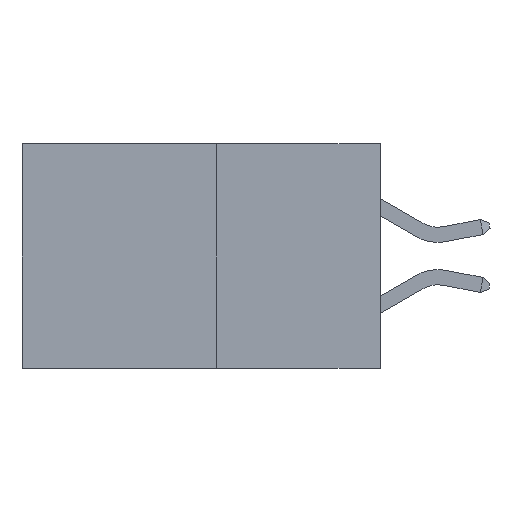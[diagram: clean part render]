
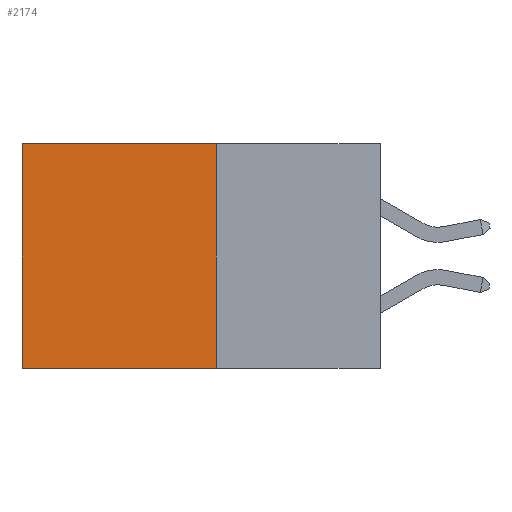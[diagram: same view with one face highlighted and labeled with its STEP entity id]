
A CAD part, left-side view. The second image highlights one B-rep face of the part: STEP entity #2174.
In plain terms, the highlighted planar face has unit normal (-1, 0, 0).
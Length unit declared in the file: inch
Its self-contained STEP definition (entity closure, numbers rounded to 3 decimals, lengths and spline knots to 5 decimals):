
#420 = LINE ( 'NONE', #1278, #32163 ) ;
#1046 = EDGE_CURVE ( 'NONE', #8502, #1778, #3159, .T. ) ;
#1087 = ORIENTED_EDGE ( 'NONE', *, *, #10690, .F. ) ;
#1278 = CARTESIAN_POINT ( 'NONE',  ( 0.277, 0.27, -0.37 ) ) ;
#1484 = PLANE ( 'NONE',  #13002 ) ;
#1778 = VERTEX_POINT ( 'NONE', #25335 ) ;
#2174 = ADVANCED_FACE ( 'NONE', ( #19634 ), #1484, .F. ) ;
#2324 = CARTESIAN_POINT ( 'NONE',  ( 0.277, 0.27, -0.37 ) ) ;
#3159 = LINE ( 'NONE', #20401, #12283 ) ;
#4904 = VECTOR ( 'NONE', #17409, 39.37008 ) ;
#6330 = ORIENTED_EDGE ( 'NONE', *, *, #1046, .T. ) ;
#8502 = VERTEX_POINT ( 'NONE', #27455 ) ;
#8801 = ORIENTED_EDGE ( 'NONE', *, *, #24155, .T. ) ;
#9324 = VECTOR ( 'NONE', #13642, 39.37008 ) ;
#10690 = EDGE_CURVE ( 'NONE', #8502, #12265, #420, .T. ) ;
#11137 = CARTESIAN_POINT ( 'NONE',  ( 0.277, 0.59, -0.37 ) ) ;
#12265 = VERTEX_POINT ( 'NONE', #29933 ) ;
#12283 = VECTOR ( 'NONE', #19959, 39.37008 ) ;
#13002 = AXIS2_PLACEMENT_3D ( 'NONE', #16773, #32307, #31680 ) ;
#13642 = DIRECTION ( 'NONE',  ( 0., 0., -1. ) ) ;
#15832 = ORIENTED_EDGE ( 'NONE', *, *, #20742, .F. ) ;
#16773 = CARTESIAN_POINT ( 'NONE',  ( 0.277, 0.27, -0.37 ) ) ;
#17409 = DIRECTION ( 'NONE',  ( 0., 1., 0. ) ) ;
#17697 = VERTEX_POINT ( 'NONE', #18727 ) ;
#18727 = CARTESIAN_POINT ( 'NONE',  ( 0.277, 0.59, -0.37 ) ) ;
#19634 = FACE_OUTER_BOUND ( 'NONE', #28226, .T. ) ;
#19959 = DIRECTION ( 'NONE',  ( 0., 1., 0. ) ) ;
#20401 = CARTESIAN_POINT ( 'NONE',  ( 0.277, 0.27, 0. ) ) ;
#20742 = EDGE_CURVE ( 'NONE', #12265, #17697, #24153, .T. ) ;
#21435 = DIRECTION ( 'NONE',  ( 0., 0., -1. ) ) ;
#24153 = LINE ( 'NONE', #2324, #4904 ) ;
#24155 = EDGE_CURVE ( 'NONE', #1778, #17697, #29280, .T. ) ;
#25335 = CARTESIAN_POINT ( 'NONE',  ( 0.277, 0.59, 0. ) ) ;
#27455 = CARTESIAN_POINT ( 'NONE',  ( 0.277, 0.27, 0. ) ) ;
#28226 = EDGE_LOOP ( 'NONE', ( #8801, #15832, #1087, #6330 ) ) ;
#29280 = LINE ( 'NONE', #11137, #9324 ) ;
#29933 = CARTESIAN_POINT ( 'NONE',  ( 0.277, 0.27, -0.37 ) ) ;
#31680 = DIRECTION ( 'NONE',  ( 0., 0., -1. ) ) ;
#32163 = VECTOR ( 'NONE', #21435, 39.37008 ) ;
#32307 = DIRECTION ( 'NONE',  ( 1., 0., 0. ) ) ;
